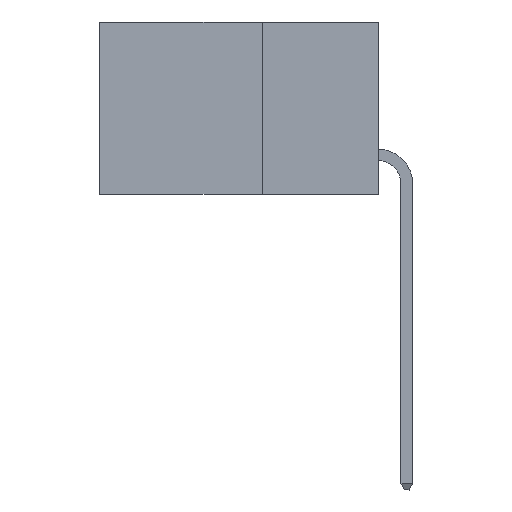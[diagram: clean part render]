
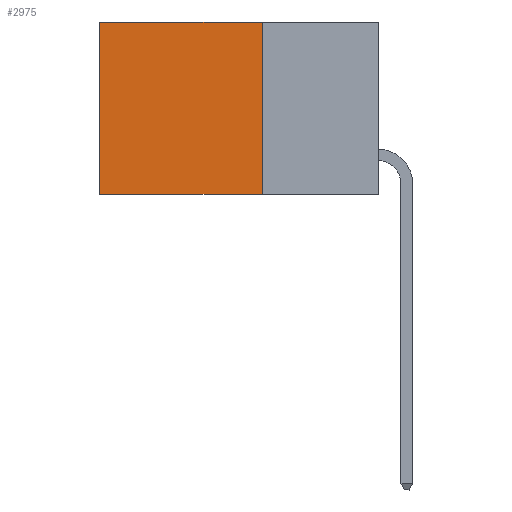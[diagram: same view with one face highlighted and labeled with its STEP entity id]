
A CAD part, left-side view. The second image highlights one B-rep face of the part: STEP entity #2975.
In plain terms, the highlighted planar face has unit normal (-1, 0, 0).
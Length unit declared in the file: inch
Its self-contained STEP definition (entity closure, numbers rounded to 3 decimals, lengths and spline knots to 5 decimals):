
#444 = CARTESIAN_POINT ( 'NONE',  ( 0.298, 0.6, 0. ) ) ;
#786 = VERTEX_POINT ( 'NONE', #444 ) ;
#919 = AXIS2_PLACEMENT_3D ( 'NONE', #10050, #3446, #10084 ) ;
#1074 = LINE ( 'NONE', #1702, #3667 ) ;
#1448 = CARTESIAN_POINT ( 'NONE',  ( 0.298, 0.25, 0. ) ) ;
#1537 = ORIENTED_EDGE ( 'NONE', *, *, #2685, .F. ) ;
#1653 = VERTEX_POINT ( 'NONE', #10859 ) ;
#1702 = CARTESIAN_POINT ( 'NONE',  ( 0.298, 0.6, 0. ) ) ;
#1826 = DIRECTION ( 'NONE',  ( 0., 0., -1. ) ) ;
#2122 = VERTEX_POINT ( 'NONE', #7094 ) ;
#2418 = VECTOR ( 'NONE', #1826, 39.37008 ) ;
#2685 = EDGE_CURVE ( 'NONE', #9072, #1653, #11598, .T. ) ;
#2975 = ADVANCED_FACE ( 'NONE', ( #9337 ), #7296, .F. ) ;
#3276 = LINE ( 'NONE', #9734, #8285 ) ;
#3446 = DIRECTION ( 'NONE',  ( 1., 0., 0. ) ) ;
#3667 = VECTOR ( 'NONE', #5429, 39.37008 ) ;
#3988 = EDGE_CURVE ( 'NONE', #786, #2122, #1074, .T. ) ;
#4539 = CARTESIAN_POINT ( 'NONE',  ( 0.298, 0.25, 0. ) ) ;
#5258 = VECTOR ( 'NONE', #10593, 39.37008 ) ;
#5429 = DIRECTION ( 'NONE',  ( 0., 0., -1. ) ) ;
#5441 = EDGE_LOOP ( 'NONE', ( #11302, #11994, #1537, #10758 ) ) ;
#6886 = CARTESIAN_POINT ( 'NONE',  ( 0.298, 0.25, 0. ) ) ;
#7094 = CARTESIAN_POINT ( 'NONE',  ( 0.298, 0.6, -0.37 ) ) ;
#7186 = EDGE_CURVE ( 'NONE', #9072, #786, #10430, .T. ) ;
#7296 = PLANE ( 'NONE',  #919 ) ;
#8285 = VECTOR ( 'NONE', #8703, 39.37008 ) ;
#8703 = DIRECTION ( 'NONE',  ( 0., 1., 0. ) ) ;
#9072 = VERTEX_POINT ( 'NONE', #1448 ) ;
#9337 = FACE_OUTER_BOUND ( 'NONE', #5441, .T. ) ;
#9734 = CARTESIAN_POINT ( 'NONE',  ( 0.298, 0.25, -0.37 ) ) ;
#10050 = CARTESIAN_POINT ( 'NONE',  ( 0.298, 0.25, 0. ) ) ;
#10084 = DIRECTION ( 'NONE',  ( 0., 0., -1. ) ) ;
#10430 = LINE ( 'NONE', #6886, #5258 ) ;
#10593 = DIRECTION ( 'NONE',  ( 0., 1., 0. ) ) ;
#10758 = ORIENTED_EDGE ( 'NONE', *, *, #7186, .T. ) ;
#10859 = CARTESIAN_POINT ( 'NONE',  ( 0.298, 0.25, -0.37 ) ) ;
#11181 = EDGE_CURVE ( 'NONE', #1653, #2122, #3276, .T. ) ;
#11302 = ORIENTED_EDGE ( 'NONE', *, *, #3988, .T. ) ;
#11598 = LINE ( 'NONE', #4539, #2418 ) ;
#11994 = ORIENTED_EDGE ( 'NONE', *, *, #11181, .F. ) ;
